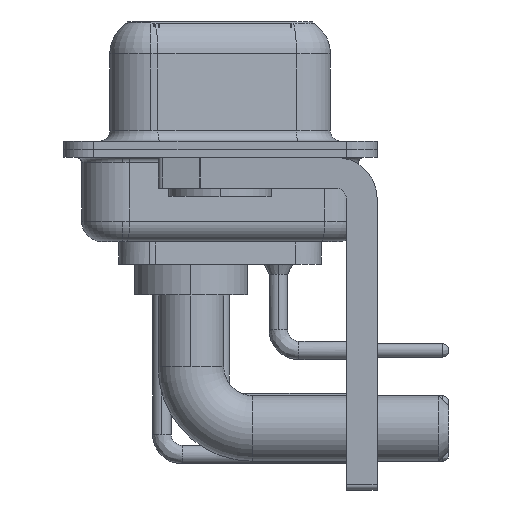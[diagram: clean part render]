
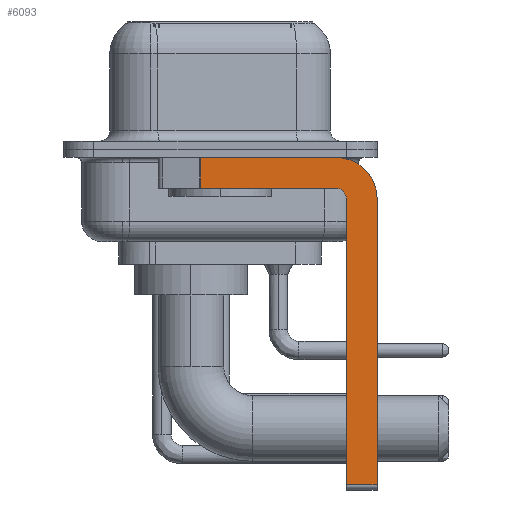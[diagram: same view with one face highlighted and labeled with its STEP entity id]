
A CAD part, left-side view. The second image highlights one B-rep face of the part: STEP entity #6093.
In plain terms, the highlighted planar face has unit normal (-1, 0, 0).
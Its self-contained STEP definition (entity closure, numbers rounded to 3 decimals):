
#1791 = CARTESIAN_POINT ( 'NONE',  ( -2.9, -7.65, -2.4 ) ) ;
#2658 = CARTESIAN_POINT ( 'NONE',  ( -2.9, -5.65, -1.9 ) ) ;
#3010 = CARTESIAN_POINT ( 'NONE',  ( -2.9, -5.65, -2.4 ) ) ;
#3284 = VERTEX_POINT ( 'NONE', #27416 ) ;
#3355 = CIRCLE ( 'NONE', #22226, 0.5 ) ;
#4067 = DIRECTION ( 'NONE',  ( 1., 0., 0. ) ) ;
#5040 = DIRECTION ( 'NONE',  ( 0., 0., 1. ) ) ;
#5173 = ORIENTED_EDGE ( 'NONE', *, *, #26002, .F. ) ;
#5407 = DIRECTION ( 'NONE',  ( 0., 0., 1. ) ) ;
#5762 = LINE ( 'NONE', #16030, #32225 ) ;
#6093 = ADVANCED_FACE ( 'NONE', ( #24591 ), #32181, .F. ) ;
#6128 = LINE ( 'NONE', #8477, #12290 ) ;
#6556 = EDGE_CURVE ( 'NONE', #19393, #20900, #22355, .T. ) ;
#7158 = AXIS2_PLACEMENT_3D ( 'NONE', #27094, #4067, #12152 ) ;
#8143 = EDGE_CURVE ( 'NONE', #17711, #33272, #18766, .T. ) ;
#8477 = CARTESIAN_POINT ( 'NONE',  ( -2.9, 0.978, -1.9 ) ) ;
#8765 = DIRECTION ( 'NONE',  ( 0., 1., 0. ) ) ;
#10076 = DIRECTION ( 'NONE',  ( 0., 0., -1. ) ) ;
#11453 = VECTOR ( 'NONE', #5040, 1000. ) ;
#12152 = DIRECTION ( 'NONE',  ( 0., 0., -1. ) ) ;
#12290 = VECTOR ( 'NONE', #21935, 1000. ) ;
#13560 = CIRCLE ( 'NONE', #32391, 2. ) ;
#14695 = VECTOR ( 'NONE', #24714, 1000. ) ;
#15637 = LINE ( 'NONE', #19899, #32489 ) ;
#15970 = DIRECTION ( 'NONE',  ( 1., 0., 0. ) ) ;
#16030 = CARTESIAN_POINT ( 'NONE',  ( -2.9, -5.65, -1.9 ) ) ;
#16308 = CARTESIAN_POINT ( 'NONE',  ( -2.9, -5.65, -0.4 ) ) ;
#17074 = VERTEX_POINT ( 'NONE', #25449 ) ;
#17112 = EDGE_LOOP ( 'NONE', ( #20734, #24697, #21629, #5173, #25679, #30424, #26170, #28020 ) ) ;
#17711 = VERTEX_POINT ( 'NONE', #1791 ) ;
#17843 = LINE ( 'NONE', #23377, #11453 ) ;
#18766 = LINE ( 'NONE', #26312, #23862 ) ;
#19290 = CARTESIAN_POINT ( 'NONE',  ( -2.9, 0.978, -0.4 ) ) ;
#19393 = VERTEX_POINT ( 'NONE', #19290 ) ;
#19684 = CARTESIAN_POINT ( 'NONE',  ( -2.9, 3., -0.4 ) ) ;
#19899 = CARTESIAN_POINT ( 'NONE',  ( -2.9, -5.65, -16.35 ) ) ;
#20711 = EDGE_CURVE ( 'NONE', #17074, #32878, #17843, .T. ) ;
#20734 = ORIENTED_EDGE ( 'NONE', *, *, #6556, .F. ) ;
#20900 = VERTEX_POINT ( 'NONE', #16308 ) ;
#21358 = EDGE_CURVE ( 'NONE', #19393, #3284, #6128, .T. ) ;
#21629 = ORIENTED_EDGE ( 'NONE', *, *, #21851, .F. ) ;
#21851 = EDGE_CURVE ( 'NONE', #22537, #3284, #5762, .T. ) ;
#21935 = DIRECTION ( 'NONE',  ( 0., 0., -1. ) ) ;
#22226 = AXIS2_PLACEMENT_3D ( 'NONE', #25753, #23236, #5407 ) ;
#22273 = CARTESIAN_POINT ( 'NONE',  ( -2.9, -7.65, -16.35 ) ) ;
#22355 = LINE ( 'NONE', #19684, #14695 ) ;
#22537 = VERTEX_POINT ( 'NONE', #2658 ) ;
#23236 = DIRECTION ( 'NONE',  ( -1., 0., 0. ) ) ;
#23300 = CARTESIAN_POINT ( 'NONE',  ( -2.9, -6.15, -2.4 ) ) ;
#23377 = CARTESIAN_POINT ( 'NONE',  ( -2.9, -6.15, -16.6 ) ) ;
#23862 = VECTOR ( 'NONE', #10076, 1000. ) ;
#24591 = FACE_OUTER_BOUND ( 'NONE', #17112, .T. ) ;
#24697 = ORIENTED_EDGE ( 'NONE', *, *, #21358, .T. ) ;
#24714 = DIRECTION ( 'NONE',  ( 0., -1., 0. ) ) ;
#24754 = EDGE_CURVE ( 'NONE', #20900, #17711, #13560, .T. ) ;
#25449 = CARTESIAN_POINT ( 'NONE',  ( -2.9, -6.15, -16.35 ) ) ;
#25679 = ORIENTED_EDGE ( 'NONE', *, *, #20711, .F. ) ;
#25705 = DIRECTION ( 'NONE',  ( 0., -1., 0. ) ) ;
#25753 = CARTESIAN_POINT ( 'NONE',  ( -2.9, -5.65, -2.4 ) ) ;
#26002 = EDGE_CURVE ( 'NONE', #32878, #22537, #3355, .T. ) ;
#26170 = ORIENTED_EDGE ( 'NONE', *, *, #8143, .F. ) ;
#26312 = CARTESIAN_POINT ( 'NONE',  ( -2.9, -7.65, -2.4 ) ) ;
#27094 = CARTESIAN_POINT ( 'NONE',  ( -2.9, -5.65, -2.4 ) ) ;
#27416 = CARTESIAN_POINT ( 'NONE',  ( -2.9, 0.978, -1.9 ) ) ;
#27602 = EDGE_CURVE ( 'NONE', #17074, #33272, #15637, .T. ) ;
#28020 = ORIENTED_EDGE ( 'NONE', *, *, #24754, .F. ) ;
#28727 = DIRECTION ( 'NONE',  ( 0., 0., -1. ) ) ;
#30424 = ORIENTED_EDGE ( 'NONE', *, *, #27602, .T. ) ;
#32181 = PLANE ( 'NONE',  #7158 ) ;
#32225 = VECTOR ( 'NONE', #8765, 1000. ) ;
#32391 = AXIS2_PLACEMENT_3D ( 'NONE', #3010, #15970, #28727 ) ;
#32489 = VECTOR ( 'NONE', #25705, 1000. ) ;
#32878 = VERTEX_POINT ( 'NONE', #23300 ) ;
#33272 = VERTEX_POINT ( 'NONE', #22273 ) ;
